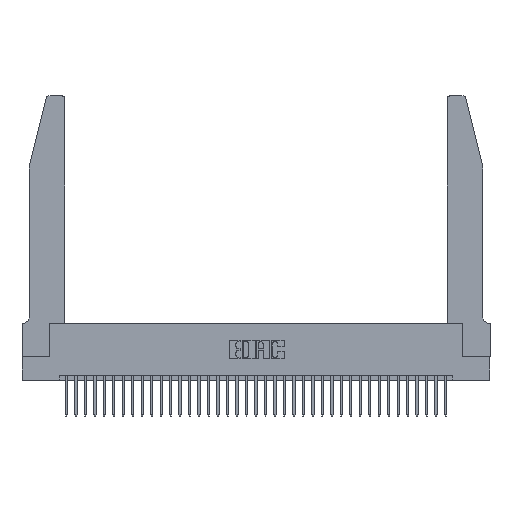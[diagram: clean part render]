
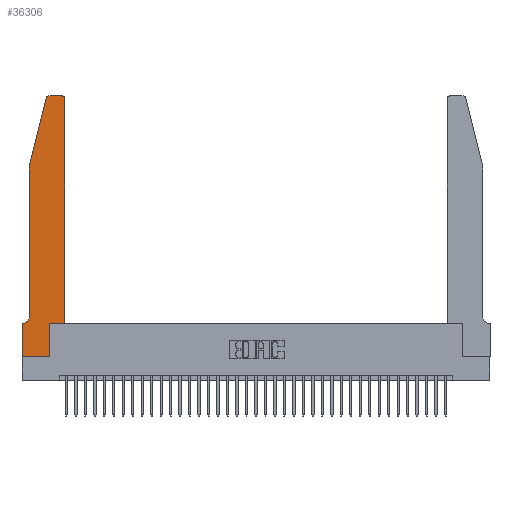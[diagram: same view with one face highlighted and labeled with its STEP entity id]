
A CAD part, top view. The second image highlights one B-rep face of the part: STEP entity #36306.
In plain terms, the highlighted planar face has unit normal (0, 0, 1).
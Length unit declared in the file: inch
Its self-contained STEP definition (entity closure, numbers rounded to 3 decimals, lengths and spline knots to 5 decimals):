
#55 = CARTESIAN_POINT ( 'NONE',  ( 0.0055, 0.42, 0.37 ) ) ;
#206 = VERTEX_POINT ( 'NONE', #32156 ) ;
#464 = CARTESIAN_POINT ( 'NONE',  ( 0., 0.35, 0.37 ) ) ;
#967 = CARTESIAN_POINT ( 'NONE',  ( 0.0755, 2., 0.37 ) ) ;
#2124 = LINE ( 'NONE', #4567, #26368 ) ;
#2248 = CARTESIAN_POINT ( 'NONE',  ( 0.4505, 2.72, 0.37 ) ) ;
#2254 = CIRCLE ( 'NONE', #35778, 0.07 ) ;
#2452 = CARTESIAN_POINT ( 'NONE',  ( 0.4205, 2.72, 0.37 ) ) ;
#2580 = DIRECTION ( 'NONE',  ( 0., 0., 1. ) ) ;
#2928 = ORIENTED_EDGE ( 'NONE', *, *, #8192, .T. ) ;
#2990 = CARTESIAN_POINT ( 'NONE',  ( 0., 0., 0.37 ) ) ;
#3698 = CARTESIAN_POINT ( 'NONE',  ( 0.4505, 0.35, 0.37 ) ) ;
#3834 = EDGE_CURVE ( 'NONE', #24300, #32169, #36131, .T. ) ;
#3859 = ORIENTED_EDGE ( 'NONE', *, *, #18390, .T. ) ;
#3896 = DIRECTION ( 'NONE',  ( -0.239, -0.971, 0. ) ) ;
#4380 = CARTESIAN_POINT ( 'NONE',  ( 0., 0., 0.37 ) ) ;
#4515 = CARTESIAN_POINT ( 'NONE',  ( 0.0755, 0.35, 0.37 ) ) ;
#4567 = CARTESIAN_POINT ( 'NONE',  ( 0.2865, 0.35, 0.37 ) ) ;
#4774 = LINE ( 'NONE', #3698, #16876 ) ;
#5609 = ORIENTED_EDGE ( 'NONE', *, *, #17092, .T. ) ;
#5754 = CARTESIAN_POINT ( 'NONE',  ( 0.0755, 2., 0.37 ) ) ;
#6351 = DIRECTION ( 'NONE',  ( 0., 0., -1. ) ) ;
#7204 = EDGE_CURVE ( 'NONE', #25189, #206, #2254, .T. ) ;
#8192 = EDGE_CURVE ( 'NONE', #29467, #25189, #22820, .T. ) ;
#9094 = EDGE_CURVE ( 'NONE', #22013, #29068, #34380, .T. ) ;
#9467 = DIRECTION ( 'NONE',  ( -1., 0., 0. ) ) ;
#9669 = CARTESIAN_POINT ( 'NONE',  ( 0.4505, 0.35, 0.37 ) ) ;
#9848 = EDGE_LOOP ( 'NONE', ( #10855, #9963, #3859, #2928, #23021, #23617, #33035, #29127, #10611, #33163, #24980, #5609 ) ) ;
#9963 = ORIENTED_EDGE ( 'NONE', *, *, #9094, .T. ) ;
#10134 = DIRECTION ( 'NONE',  ( 0., -1., 0. ) ) ;
#10355 = DIRECTION ( 'NONE',  ( 1., 0., 0. ) ) ;
#10611 = ORIENTED_EDGE ( 'NONE', *, *, #31642, .T. ) ;
#10855 = ORIENTED_EDGE ( 'NONE', *, *, #12913, .T. ) ;
#10876 = CARTESIAN_POINT ( 'NONE',  ( 0.2605, 2.75, 0.37 ) ) ;
#11409 = EDGE_CURVE ( 'NONE', #32169, #22810, #4774, .T. ) ;
#11961 = CARTESIAN_POINT ( 'NONE',  ( 0.284, 2.72, 0.37 ) ) ;
#12913 = EDGE_CURVE ( 'NONE', #29561, #22013, #36837, .T. ) ;
#14042 = EDGE_CURVE ( 'NONE', #206, #14382, #18920, .T. ) ;
#14382 = VERTEX_POINT ( 'NONE', #20914 ) ;
#14485 = CARTESIAN_POINT ( 'NONE',  ( 0., 0., 0.37 ) ) ;
#14495 = VERTEX_POINT ( 'NONE', #15884 ) ;
#14524 = DIRECTION ( 'NONE',  ( 1., 0., 0. ) ) ;
#14953 = PLANE ( 'NONE',  #19077 ) ;
#15884 = CARTESIAN_POINT ( 'NONE',  ( 0.2865, 0., 0.37 ) ) ;
#16748 = EDGE_CURVE ( 'NONE', #14382, #31956, #22718, .T. ) ;
#16876 = VECTOR ( 'NONE', #23620, 39.37008 ) ;
#16882 = DIRECTION ( 'NONE',  ( 1., 0., 0. ) ) ;
#17092 = EDGE_CURVE ( 'NONE', #22810, #29561, #31579, .T. ) ;
#17659 = VECTOR ( 'NONE', #22510, 39.37008 ) ;
#18261 = LINE ( 'NONE', #2990, #20065 ) ;
#18390 = EDGE_CURVE ( 'NONE', #29068, #29467, #19043, .T. ) ;
#18920 = LINE ( 'NONE', #4515, #24673 ) ;
#19043 = LINE ( 'NONE', #967, #26650 ) ;
#19077 = AXIS2_PLACEMENT_3D ( 'NONE', #464, #20582, #23326 ) ;
#20065 = VECTOR ( 'NONE', #34270, 39.37008 ) ;
#20582 = DIRECTION ( 'NONE',  ( 0., 0., 1. ) ) ;
#20914 = CARTESIAN_POINT ( 'NONE',  ( 0., 0.35, 0.37 ) ) ;
#22013 = VERTEX_POINT ( 'NONE', #36059 ) ;
#22510 = DIRECTION ( 'NONE',  ( -1., 0., 0. ) ) ;
#22524 = DIRECTION ( 'NONE',  ( 0., 0., 1. ) ) ;
#22718 = LINE ( 'NONE', #4380, #36103 ) ;
#22810 = VERTEX_POINT ( 'NONE', #2248 ) ;
#22820 = LINE ( 'NONE', #5754, #33078 ) ;
#23021 = ORIENTED_EDGE ( 'NONE', *, *, #7204, .T. ) ;
#23189 = DIRECTION ( 'NONE',  ( 0., -1., 0. ) ) ;
#23226 = CARTESIAN_POINT ( 'NONE',  ( 0.4205, 2.75, 0.37 ) ) ;
#23326 = DIRECTION ( 'NONE',  ( 1., 0., 0. ) ) ;
#23617 = ORIENTED_EDGE ( 'NONE', *, *, #14042, .T. ) ;
#23620 = DIRECTION ( 'NONE',  ( 0., 1., 0. ) ) ;
#24300 = VERTEX_POINT ( 'NONE', #26222 ) ;
#24472 = CARTESIAN_POINT ( 'NONE',  ( 0.0755, 0.42, 0.37 ) ) ;
#24673 = VECTOR ( 'NONE', #36753, 39.37008 ) ;
#24693 = FACE_OUTER_BOUND ( 'NONE', #9848, .T. ) ;
#24980 = ORIENTED_EDGE ( 'NONE', *, *, #11409, .T. ) ;
#25189 = VERTEX_POINT ( 'NONE', #24472 ) ;
#26222 = CARTESIAN_POINT ( 'NONE',  ( 0.2865, 0.35, 0.37 ) ) ;
#26368 = VECTOR ( 'NONE', #30057, 39.37008 ) ;
#26475 = AXIS2_PLACEMENT_3D ( 'NONE', #11961, #2580, #14524 ) ;
#26650 = VECTOR ( 'NONE', #3896, 39.37008 ) ;
#27628 = VECTOR ( 'NONE', #10355, 39.37008 ) ;
#28175 = CARTESIAN_POINT ( 'NONE',  ( 0.0755, 2., 0.37 ) ) ;
#29068 = VERTEX_POINT ( 'NONE', #32459 ) ;
#29127 = ORIENTED_EDGE ( 'NONE', *, *, #32635, .T. ) ;
#29467 = VERTEX_POINT ( 'NONE', #28175 ) ;
#29561 = VERTEX_POINT ( 'NONE', #23226 ) ;
#30057 = DIRECTION ( 'NONE',  ( 0., 1., 0. ) ) ;
#31579 = CIRCLE ( 'NONE', #32276, 0.03 ) ;
#31642 = EDGE_CURVE ( 'NONE', #14495, #24300, #2124, .T. ) ;
#31956 = VERTEX_POINT ( 'NONE', #14485 ) ;
#32156 = CARTESIAN_POINT ( 'NONE',  ( 0.0055, 0.35, 0.37 ) ) ;
#32169 = VERTEX_POINT ( 'NONE', #9669 ) ;
#32276 = AXIS2_PLACEMENT_3D ( 'NONE', #2452, #22524, #16882 ) ;
#32459 = CARTESIAN_POINT ( 'NONE',  ( 0.25487, 2.72718, 0.37 ) ) ;
#32635 = EDGE_CURVE ( 'NONE', #31956, #14495, #18261, .T. ) ;
#33035 = ORIENTED_EDGE ( 'NONE', *, *, #16748, .T. ) ;
#33078 = VECTOR ( 'NONE', #23189, 39.37008 ) ;
#33163 = ORIENTED_EDGE ( 'NONE', *, *, #3834, .T. ) ;
#34270 = DIRECTION ( 'NONE',  ( 1., 0., 0. ) ) ;
#34380 = CIRCLE ( 'NONE', #26475, 0.03 ) ;
#35778 = AXIS2_PLACEMENT_3D ( 'NONE', #55, #6351, #9467 ) ;
#36059 = CARTESIAN_POINT ( 'NONE',  ( 0.284, 2.75, 0.37 ) ) ;
#36103 = VECTOR ( 'NONE', #10134, 39.37008 ) ;
#36131 = LINE ( 'NONE', #36479, #27628 ) ;
#36306 = ADVANCED_FACE ( 'NONE', ( #24693 ), #14953, .T. ) ;
#36479 = CARTESIAN_POINT ( 'NONE',  ( 0.4505, 0.35, 0.37 ) ) ;
#36753 = DIRECTION ( 'NONE',  ( -1., 0., 0. ) ) ;
#36837 = LINE ( 'NONE', #10876, #17659 ) ;
